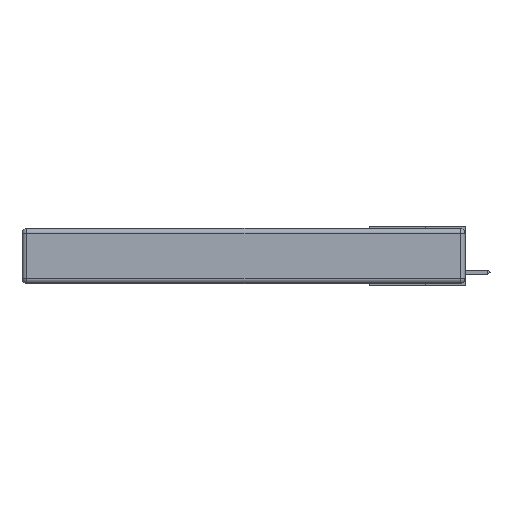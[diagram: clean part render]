
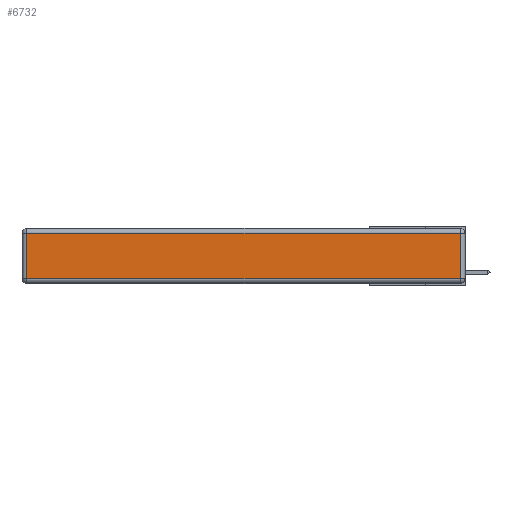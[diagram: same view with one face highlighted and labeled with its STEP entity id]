
A CAD part, left-side view. The second image highlights one B-rep face of the part: STEP entity #6732.
In plain terms, the highlighted planar face has unit normal (-1, 0, 0).
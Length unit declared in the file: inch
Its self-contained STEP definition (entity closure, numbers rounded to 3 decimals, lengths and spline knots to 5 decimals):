
#16 = VERTEX_POINT ( 'NONE', #5301 ) ;
#359 = DIRECTION ( 'NONE',  ( 0., 0., 1. ) ) ;
#1120 = VERTEX_POINT ( 'NONE', #11002 ) ;
#2512 = ORIENTED_EDGE ( 'NONE', *, *, #5936, .T. ) ;
#2990 = LINE ( 'NONE', #11295, #3570 ) ;
#3570 = VECTOR ( 'NONE', #6721, 39.37008 ) ;
#4261 = VERTEX_POINT ( 'NONE', #10608 ) ;
#4850 = EDGE_CURVE ( 'NONE', #16, #1120, #2990, .T. ) ;
#4997 = CARTESIAN_POINT ( 'NONE',  ( 0., 0., -0.313 ) ) ;
#5010 = CARTESIAN_POINT ( 'NONE',  ( 0., 0.03, -0.343 ) ) ;
#5118 = CARTESIAN_POINT ( 'NONE',  ( 0., 2.75, -0.03 ) ) ;
#5203 = VECTOR ( 'NONE', #359, 39.37008 ) ;
#5301 = CARTESIAN_POINT ( 'NONE',  ( 0., 2.72, -0.03 ) ) ;
#5936 = EDGE_CURVE ( 'NONE', #7507, #4261, #15187, .T. ) ;
#6721 = DIRECTION ( 'NONE',  ( 0., 0., -1. ) ) ;
#6732 = ADVANCED_FACE ( 'NONE', ( #11220 ), #15042, .T. ) ;
#6743 = VECTOR ( 'NONE', #14732, 39.37008 ) ;
#7310 = LINE ( 'NONE', #5118, #6743 ) ;
#7330 = LINE ( 'NONE', #4997, #8451 ) ;
#7507 = VERTEX_POINT ( 'NONE', #15586 ) ;
#7915 = CARTESIAN_POINT ( 'NONE',  ( 0., 0., -0.343 ) ) ;
#8451 = VECTOR ( 'NONE', #14655, 39.37008 ) ;
#9251 = DIRECTION ( 'NONE',  ( -1., 0., 0. ) ) ;
#9263 = ORIENTED_EDGE ( 'NONE', *, *, #4850, .T. ) ;
#10527 = ORIENTED_EDGE ( 'NONE', *, *, #13042, .T. ) ;
#10608 = CARTESIAN_POINT ( 'NONE',  ( 0., 0.03, -0.03 ) ) ;
#11002 = CARTESIAN_POINT ( 'NONE',  ( 0., 2.72, -0.313 ) ) ;
#11220 = FACE_OUTER_BOUND ( 'NONE', #12356, .T. ) ;
#11295 = CARTESIAN_POINT ( 'NONE',  ( 0., 2.72, -0.343 ) ) ;
#11378 = DIRECTION ( 'NONE',  ( 0., 0., 1. ) ) ;
#11915 = EDGE_CURVE ( 'NONE', #1120, #7507, #7330, .T. ) ;
#12356 = EDGE_LOOP ( 'NONE', ( #13958, #2512, #10527, #9263 ) ) ;
#13042 = EDGE_CURVE ( 'NONE', #4261, #16, #7310, .T. ) ;
#13958 = ORIENTED_EDGE ( 'NONE', *, *, #11915, .T. ) ;
#14230 = AXIS2_PLACEMENT_3D ( 'NONE', #7915, #9251, #11378 ) ;
#14655 = DIRECTION ( 'NONE',  ( 0., -1., 0. ) ) ;
#14732 = DIRECTION ( 'NONE',  ( 0., 1., 0. ) ) ;
#15042 = PLANE ( 'NONE',  #14230 ) ;
#15187 = LINE ( 'NONE', #5010, #5203 ) ;
#15586 = CARTESIAN_POINT ( 'NONE',  ( 0., 0.03, -0.313 ) ) ;
